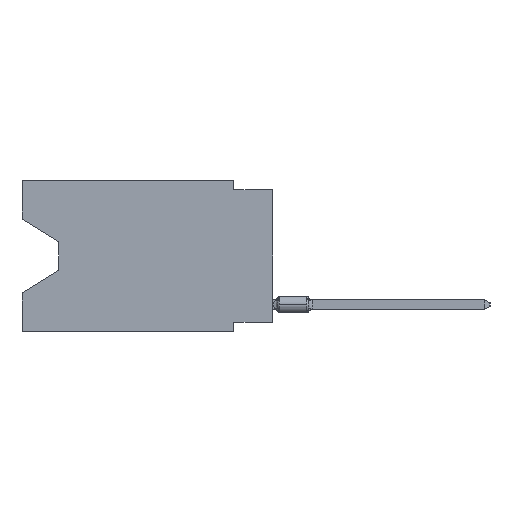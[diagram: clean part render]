
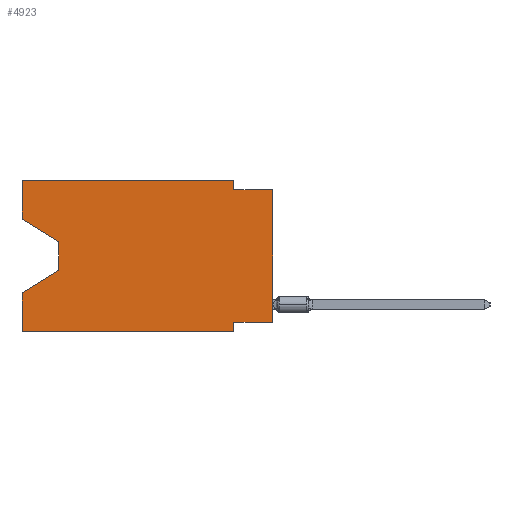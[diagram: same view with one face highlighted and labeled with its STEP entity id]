
A CAD part, left-side view. The second image highlights one B-rep face of the part: STEP entity #4923.
In plain terms, the highlighted planar face has unit normal (-1, 0, 0).
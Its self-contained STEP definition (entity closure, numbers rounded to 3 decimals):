
#284 = CARTESIAN_POINT ( 'NONE',  ( 0., 16.383, -9.906 ) ) ;
#508 = LINE ( 'NONE', #20275, #25903 ) ;
#764 = VERTEX_POINT ( 'NONE', #5841 ) ;
#1201 = CARTESIAN_POINT ( 'NONE',  ( 0., 0., -9.271 ) ) ;
#1263 = LINE ( 'NONE', #13751, #3257 ) ;
#1338 = CARTESIAN_POINT ( 'NONE',  ( 0., 2.54, -9.271 ) ) ;
#1884 = CARTESIAN_POINT ( 'NONE',  ( 0., 2.54, -9.906 ) ) ;
#2255 = CARTESIAN_POINT ( 'NONE',  ( 0., 16.383, 0. ) ) ;
#2976 = FACE_OUTER_BOUND ( 'NONE', #11191, .T. ) ;
#3169 = ORIENTED_EDGE ( 'NONE', *, *, #23630, .F. ) ;
#3216 = VECTOR ( 'NONE', #9892, 1000. ) ;
#3257 = VECTOR ( 'NONE', #6318, 1000. ) ;
#3295 = CARTESIAN_POINT ( 'NONE',  ( 0., 16.383, 0. ) ) ;
#3313 = LINE ( 'NONE', #27547, #18622 ) ;
#3844 = DIRECTION ( 'NONE',  ( 0., 0., 1. ) ) ;
#4158 = VERTEX_POINT ( 'NONE', #23890 ) ;
#4202 = ORIENTED_EDGE ( 'NONE', *, *, #4471, .F. ) ;
#4471 = EDGE_CURVE ( 'NONE', #27291, #17808, #8960, .T. ) ;
#4923 = ADVANCED_FACE ( 'NONE', ( #2976 ), #27688, .F. ) ;
#5656 = LINE ( 'NONE', #284, #27121 ) ;
#5759 = ORIENTED_EDGE ( 'NONE', *, *, #31878, .F. ) ;
#5841 = CARTESIAN_POINT ( 'NONE',  ( 0., 16.383, -9.906 ) ) ;
#6318 = DIRECTION ( 'NONE',  ( 0., 0., -1. ) ) ;
#7313 = EDGE_CURVE ( 'NONE', #764, #10838, #5656, .T. ) ;
#7515 = EDGE_CURVE ( 'NONE', #8863, #17808, #18559, .T. ) ;
#8328 = DIRECTION ( 'NONE',  ( 1., 0., 0. ) ) ;
#8863 = VERTEX_POINT ( 'NONE', #15835 ) ;
#8960 = LINE ( 'NONE', #28333, #12240 ) ;
#9061 = VECTOR ( 'NONE', #26248, 1000. ) ;
#9848 = CARTESIAN_POINT ( 'NONE',  ( 0., 0., -0.635 ) ) ;
#9892 = DIRECTION ( 'NONE',  ( 0., 0., 1. ) ) ;
#10007 = CARTESIAN_POINT ( 'NONE',  ( 0., 16.383, -7.36 ) ) ;
#10680 = DIRECTION ( 'NONE',  ( 0., -1., 0. ) ) ;
#10838 = VERTEX_POINT ( 'NONE', #29155 ) ;
#11191 = EDGE_LOOP ( 'NONE', ( #19030, #13393, #21794, #3169, #20140, #29863, #5759, #23472, #4202, #28927, #21135, #19171 ) ) ;
#11791 = VERTEX_POINT ( 'NONE', #2255 ) ;
#12145 = VECTOR ( 'NONE', #25300, 1000. ) ;
#12240 = VECTOR ( 'NONE', #28497, 1000. ) ;
#12570 = LINE ( 'NONE', #13047, #12145 ) ;
#13036 = CARTESIAN_POINT ( 'NONE',  ( 0., 2.54, -0.635 ) ) ;
#13047 = CARTESIAN_POINT ( 'NONE',  ( 0., 16.383, -2.546 ) ) ;
#13196 = EDGE_CURVE ( 'NONE', #27628, #27291, #16485, .T. ) ;
#13251 = AXIS2_PLACEMENT_3D ( 'NONE', #3295, #8328, #30112 ) ;
#13393 = ORIENTED_EDGE ( 'NONE', *, *, #27790, .T. ) ;
#13536 = LINE ( 'NONE', #1201, #9061 ) ;
#13751 = CARTESIAN_POINT ( 'NONE',  ( 0., 13.97, -4.013 ) ) ;
#14253 = VECTOR ( 'NONE', #3844, 1000. ) ;
#14499 = LINE ( 'NONE', #26584, #22629 ) ;
#14558 = CARTESIAN_POINT ( 'NONE',  ( 0., 2.54, 0. ) ) ;
#15835 = CARTESIAN_POINT ( 'NONE',  ( 0., 0., -9.271 ) ) ;
#16464 = LINE ( 'NONE', #1884, #23653 ) ;
#16485 = LINE ( 'NONE', #14558, #26280 ) ;
#17712 = DIRECTION ( 'NONE',  ( 0., 0., 1. ) ) ;
#17808 = VERTEX_POINT ( 'NONE', #9848 ) ;
#18559 = LINE ( 'NONE', #25985, #14253 ) ;
#18622 = VECTOR ( 'NONE', #17712, 1000. ) ;
#18644 = EDGE_CURVE ( 'NONE', #11791, #27628, #508, .T. ) ;
#18706 = VERTEX_POINT ( 'NONE', #21348 ) ;
#19030 = ORIENTED_EDGE ( 'NONE', *, *, #29696, .T. ) ;
#19047 = EDGE_CURVE ( 'NONE', #27387, #10838, #16464, .T. ) ;
#19056 = DIRECTION ( 'NONE',  ( 0., 0., -1. ) ) ;
#19171 = ORIENTED_EDGE ( 'NONE', *, *, #26365, .F. ) ;
#20083 = CARTESIAN_POINT ( 'NONE',  ( 0., 2.54, 0. ) ) ;
#20140 = ORIENTED_EDGE ( 'NONE', *, *, #7313, .T. ) ;
#20275 = CARTESIAN_POINT ( 'NONE',  ( 0., 16.383, 0. ) ) ;
#20740 = EDGE_CURVE ( 'NONE', #21728, #26844, #14499, .T. ) ;
#21135 = ORIENTED_EDGE ( 'NONE', *, *, #18644, .F. ) ;
#21348 = CARTESIAN_POINT ( 'NONE',  ( 0., 13.97, -4.013 ) ) ;
#21728 = VERTEX_POINT ( 'NONE', #27150 ) ;
#21794 = ORIENTED_EDGE ( 'NONE', *, *, #20740, .T. ) ;
#22147 = LINE ( 'NONE', #26664, #3216 ) ;
#22629 = VECTOR ( 'NONE', #31768, 1000. ) ;
#23472 = ORIENTED_EDGE ( 'NONE', *, *, #7515, .T. ) ;
#23630 = EDGE_CURVE ( 'NONE', #764, #26844, #3313, .T. ) ;
#23653 = VECTOR ( 'NONE', #31642, 1000. ) ;
#23890 = CARTESIAN_POINT ( 'NONE',  ( 0., 16.383, -2.546 ) ) ;
#25300 = DIRECTION ( 'NONE',  ( 0., -0.855, -0.519 ) ) ;
#25903 = VECTOR ( 'NONE', #26985, 1000. ) ;
#25985 = CARTESIAN_POINT ( 'NONE',  ( 0., 0., 0. ) ) ;
#26248 = DIRECTION ( 'NONE',  ( 0., 1., 0. ) ) ;
#26280 = VECTOR ( 'NONE', #19056, 1000. ) ;
#26365 = EDGE_CURVE ( 'NONE', #4158, #11791, #22147, .T. ) ;
#26584 = CARTESIAN_POINT ( 'NONE',  ( 0., 13.97, -5.893 ) ) ;
#26664 = CARTESIAN_POINT ( 'NONE',  ( 0., 16.383, 0. ) ) ;
#26844 = VERTEX_POINT ( 'NONE', #10007 ) ;
#26985 = DIRECTION ( 'NONE',  ( 0., -1., 0. ) ) ;
#27121 = VECTOR ( 'NONE', #10680, 1000. ) ;
#27150 = CARTESIAN_POINT ( 'NONE',  ( 0., 13.97, -5.893 ) ) ;
#27291 = VERTEX_POINT ( 'NONE', #13036 ) ;
#27387 = VERTEX_POINT ( 'NONE', #1338 ) ;
#27547 = CARTESIAN_POINT ( 'NONE',  ( 0., 16.383, 0. ) ) ;
#27628 = VERTEX_POINT ( 'NONE', #20083 ) ;
#27688 = PLANE ( 'NONE',  #13251 ) ;
#27790 = EDGE_CURVE ( 'NONE', #18706, #21728, #1263, .T. ) ;
#28333 = CARTESIAN_POINT ( 'NONE',  ( 0., 0., -0.635 ) ) ;
#28497 = DIRECTION ( 'NONE',  ( 0., -1., 0. ) ) ;
#28927 = ORIENTED_EDGE ( 'NONE', *, *, #13196, .F. ) ;
#29155 = CARTESIAN_POINT ( 'NONE',  ( 0., 2.54, -9.906 ) ) ;
#29696 = EDGE_CURVE ( 'NONE', #4158, #18706, #12570, .T. ) ;
#29863 = ORIENTED_EDGE ( 'NONE', *, *, #19047, .F. ) ;
#30112 = DIRECTION ( 'NONE',  ( 0., 0., -1. ) ) ;
#31642 = DIRECTION ( 'NONE',  ( 0., 0., -1. ) ) ;
#31768 = DIRECTION ( 'NONE',  ( 0., 0.855, -0.519 ) ) ;
#31878 = EDGE_CURVE ( 'NONE', #8863, #27387, #13536, .T. ) ;
